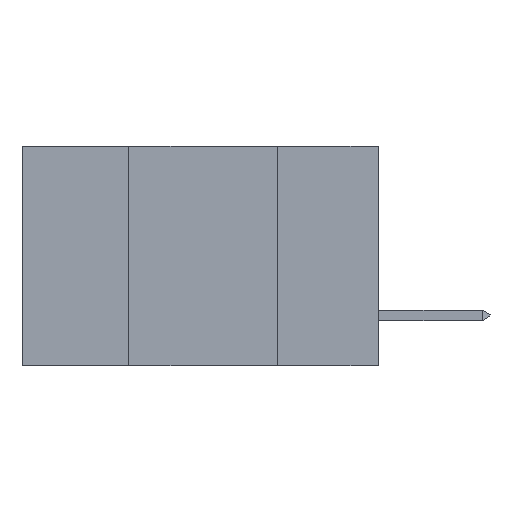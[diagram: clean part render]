
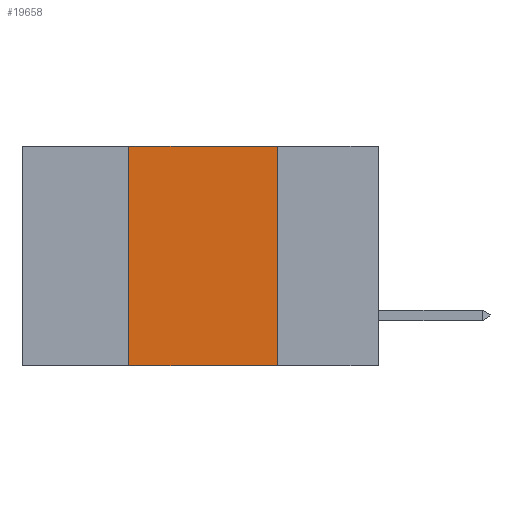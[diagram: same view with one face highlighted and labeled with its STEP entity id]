
A CAD part, left-side view. The second image highlights one B-rep face of the part: STEP entity #19658.
In plain terms, the highlighted planar face has unit normal (-1, 0, 0).
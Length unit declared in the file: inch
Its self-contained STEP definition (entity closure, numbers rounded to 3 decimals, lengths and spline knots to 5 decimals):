
#637 = VERTEX_POINT ( 'NONE', #17525 ) ;
#1853 = CARTESIAN_POINT ( 'NONE',  ( 0., 0.17, 0. ) ) ;
#2121 = LINE ( 'NONE', #21386, #21236 ) ;
#2601 = LINE ( 'NONE', #22811, #11858 ) ;
#2681 = EDGE_CURVE ( 'NONE', #6068, #637, #2121, .T. ) ;
#3517 = ORIENTED_EDGE ( 'NONE', *, *, #13148, .F. ) ;
#5184 = CARTESIAN_POINT ( 'NONE',  ( 0., 0.6, 0. ) ) ;
#6068 = VERTEX_POINT ( 'NONE', #23379 ) ;
#6842 = VECTOR ( 'NONE', #10427, 39.37008 ) ;
#6923 = PLANE ( 'NONE',  #20785 ) ;
#7396 = ORIENTED_EDGE ( 'NONE', *, *, #24389, .F. ) ;
#7644 = LINE ( 'NONE', #21667, #6842 ) ;
#7959 = VERTEX_POINT ( 'NONE', #1853 ) ;
#9234 = VERTEX_POINT ( 'NONE', #20722 ) ;
#9485 = FACE_OUTER_BOUND ( 'NONE', #16552, .T. ) ;
#9927 = DIRECTION ( 'NONE',  ( 0., 0., 1. ) ) ;
#10427 = DIRECTION ( 'NONE',  ( 0., -1., 0. ) ) ;
#11858 = VECTOR ( 'NONE', #24700, 39.37008 ) ;
#12621 = DIRECTION ( 'NONE',  ( 1., 0., 0. ) ) ;
#12861 = EDGE_CURVE ( 'NONE', #6068, #9234, #2601, .T. ) ;
#13148 = EDGE_CURVE ( 'NONE', #7959, #9234, #14861, .T. ) ;
#14173 = CARTESIAN_POINT ( 'NONE',  ( 0., 0.17, 0. ) ) ;
#14861 = LINE ( 'NONE', #14173, #23814 ) ;
#16552 = EDGE_LOOP ( 'NONE', ( #3517, #7396, #18017, #23965 ) ) ;
#17525 = CARTESIAN_POINT ( 'NONE',  ( 0., 0.42, 0. ) ) ;
#18017 = ORIENTED_EDGE ( 'NONE', *, *, #2681, .F. ) ;
#18638 = DIRECTION ( 'NONE',  ( 0., 0., -1. ) ) ;
#19658 = ADVANCED_FACE ( 'NONE', ( #9485 ), #6923, .F. ) ;
#20722 = CARTESIAN_POINT ( 'NONE',  ( 0., 0.17, -0.37 ) ) ;
#20785 = AXIS2_PLACEMENT_3D ( 'NONE', #5184, #12621, #18638 ) ;
#21236 = VECTOR ( 'NONE', #9927, 39.37008 ) ;
#21386 = CARTESIAN_POINT ( 'NONE',  ( 0., 0.42, 0. ) ) ;
#21667 = CARTESIAN_POINT ( 'NONE',  ( 0., 0.6, 0. ) ) ;
#22811 = CARTESIAN_POINT ( 'NONE',  ( 0., 0.6, -0.37 ) ) ;
#23379 = CARTESIAN_POINT ( 'NONE',  ( 0., 0.42, -0.37 ) ) ;
#23604 = DIRECTION ( 'NONE',  ( 0., 0., -1. ) ) ;
#23814 = VECTOR ( 'NONE', #23604, 39.37008 ) ;
#23965 = ORIENTED_EDGE ( 'NONE', *, *, #12861, .T. ) ;
#24389 = EDGE_CURVE ( 'NONE', #637, #7959, #7644, .T. ) ;
#24700 = DIRECTION ( 'NONE',  ( 0., -1., 0. ) ) ;
